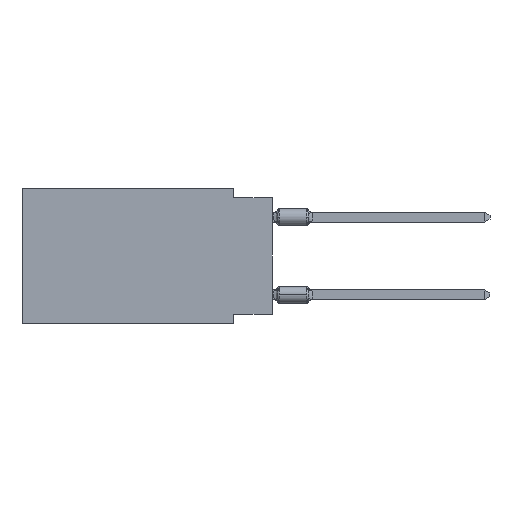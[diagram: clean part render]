
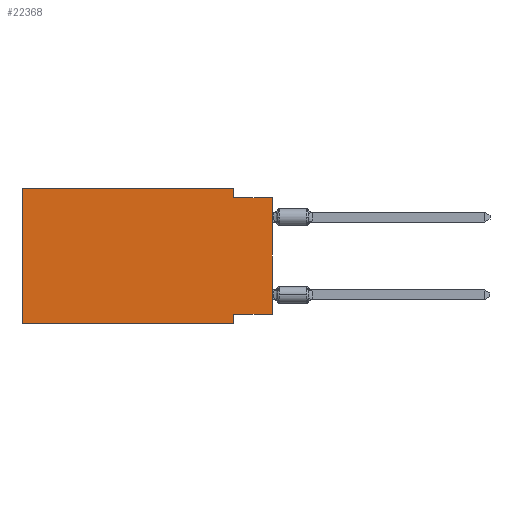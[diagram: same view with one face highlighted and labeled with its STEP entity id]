
A CAD part, left-side view. The second image highlights one B-rep face of the part: STEP entity #22368.
In plain terms, the highlighted planar face has unit normal (-1, 0, 0).
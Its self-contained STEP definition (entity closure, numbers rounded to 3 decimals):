
#188 = DIRECTION ( 'NONE',  ( 0., 0., 1. ) ) ;
#554 = PLANE ( 'NONE',  #14578 ) ;
#689 = CARTESIAN_POINT ( 'NONE',  ( 0., 16.383, -8.89 ) ) ;
#827 = ORIENTED_EDGE ( 'NONE', *, *, #16635, .F. ) ;
#1138 = DIRECTION ( 'NONE',  ( 0., -1., 0. ) ) ;
#1493 = VECTOR ( 'NONE', #17052, 1000. ) ;
#1579 = CARTESIAN_POINT ( 'NONE',  ( 0., 16.383, 0. ) ) ;
#1986 = ORIENTED_EDGE ( 'NONE', *, *, #21141, .F. ) ;
#2178 = FACE_OUTER_BOUND ( 'NONE', #10712, .T. ) ;
#2858 = ORIENTED_EDGE ( 'NONE', *, *, #10344, .F. ) ;
#2995 = EDGE_CURVE ( 'NONE', #13982, #20071, #6678, .T. ) ;
#3423 = VECTOR ( 'NONE', #1138, 1000. ) ;
#3777 = CARTESIAN_POINT ( 'NONE',  ( 0., 0., -8.255 ) ) ;
#3821 = DIRECTION ( 'NONE',  ( 1., 0., 0. ) ) ;
#3848 = CARTESIAN_POINT ( 'NONE',  ( 0., 2.54, -8.89 ) ) ;
#3850 = EDGE_CURVE ( 'NONE', #12104, #13905, #4719, .T. ) ;
#3902 = DIRECTION ( 'NONE',  ( 0., 0., 1. ) ) ;
#4116 = VECTOR ( 'NONE', #3902, 1000. ) ;
#4665 = LINE ( 'NONE', #18577, #15156 ) ;
#4695 = CARTESIAN_POINT ( 'NONE',  ( 0., 2.54, 0. ) ) ;
#4719 = LINE ( 'NONE', #20967, #14611 ) ;
#5555 = ORIENTED_EDGE ( 'NONE', *, *, #21640, .F. ) ;
#6438 = LINE ( 'NONE', #10158, #1493 ) ;
#6678 = LINE ( 'NONE', #17410, #22055 ) ;
#7951 = ORIENTED_EDGE ( 'NONE', *, *, #3850, .T. ) ;
#8048 = VERTEX_POINT ( 'NONE', #12262 ) ;
#8264 = CARTESIAN_POINT ( 'NONE',  ( 0., 0., -0.635 ) ) ;
#8575 = DIRECTION ( 'NONE',  ( 0., -1., 0. ) ) ;
#9146 = LINE ( 'NONE', #3777, #13728 ) ;
#9916 = DIRECTION ( 'NONE',  ( 0., 0., -1. ) ) ;
#10002 = LINE ( 'NONE', #8264, #3423 ) ;
#10158 = CARTESIAN_POINT ( 'NONE',  ( 0., 2.54, -8.89 ) ) ;
#10344 = EDGE_CURVE ( 'NONE', #20071, #12624, #4665, .T. ) ;
#10712 = EDGE_LOOP ( 'NONE', ( #11219, #827, #2858, #13090, #1986, #7951, #5555, #19471 ) ) ;
#10894 = DIRECTION ( 'NONE',  ( 0., 1., 0. ) ) ;
#10935 = DIRECTION ( 'NONE',  ( 0., 0., -1. ) ) ;
#11154 = EDGE_CURVE ( 'NONE', #11251, #8048, #9146, .T. ) ;
#11219 = ORIENTED_EDGE ( 'NONE', *, *, #22249, .T. ) ;
#11251 = VERTEX_POINT ( 'NONE', #11814 ) ;
#11814 = CARTESIAN_POINT ( 'NONE',  ( 0., 0., -8.255 ) ) ;
#12104 = VERTEX_POINT ( 'NONE', #689 ) ;
#12262 = CARTESIAN_POINT ( 'NONE',  ( 0., 2.54, -8.255 ) ) ;
#12624 = VERTEX_POINT ( 'NONE', #19704 ) ;
#12801 = LINE ( 'NONE', #21813, #16434 ) ;
#13090 = ORIENTED_EDGE ( 'NONE', *, *, #2995, .F. ) ;
#13728 = VECTOR ( 'NONE', #10894, 1000. ) ;
#13905 = VERTEX_POINT ( 'NONE', #3848 ) ;
#13982 = VERTEX_POINT ( 'NONE', #1579 ) ;
#14578 = AXIS2_PLACEMENT_3D ( 'NONE', #19829, #3821, #10935 ) ;
#14611 = VECTOR ( 'NONE', #8575, 1000. ) ;
#14754 = CARTESIAN_POINT ( 'NONE',  ( 0., 16.383, 0. ) ) ;
#14899 = CARTESIAN_POINT ( 'NONE',  ( 0., 0., -0.635 ) ) ;
#15156 = VECTOR ( 'NONE', #9916, 1000. ) ;
#16434 = VECTOR ( 'NONE', #188, 1000. ) ;
#16635 = EDGE_CURVE ( 'NONE', #12624, #18097, #10002, .T. ) ;
#17052 = DIRECTION ( 'NONE',  ( 0., 0., -1. ) ) ;
#17071 = DIRECTION ( 'NONE',  ( 0., -1., 0. ) ) ;
#17410 = CARTESIAN_POINT ( 'NONE',  ( 0., 16.383, 0. ) ) ;
#18097 = VERTEX_POINT ( 'NONE', #14899 ) ;
#18577 = CARTESIAN_POINT ( 'NONE',  ( 0., 2.54, 0. ) ) ;
#19471 = ORIENTED_EDGE ( 'NONE', *, *, #11154, .F. ) ;
#19704 = CARTESIAN_POINT ( 'NONE',  ( 0., 2.54, -0.635 ) ) ;
#19829 = CARTESIAN_POINT ( 'NONE',  ( 0., 16.383, 0. ) ) ;
#20071 = VERTEX_POINT ( 'NONE', #4695 ) ;
#20967 = CARTESIAN_POINT ( 'NONE',  ( 0., 16.383, -8.89 ) ) ;
#21141 = EDGE_CURVE ( 'NONE', #12104, #13982, #22139, .T. ) ;
#21640 = EDGE_CURVE ( 'NONE', #8048, #13905, #6438, .T. ) ;
#21813 = CARTESIAN_POINT ( 'NONE',  ( 0., 0., 0. ) ) ;
#22055 = VECTOR ( 'NONE', #17071, 1000. ) ;
#22139 = LINE ( 'NONE', #14754, #4116 ) ;
#22249 = EDGE_CURVE ( 'NONE', #11251, #18097, #12801, .T. ) ;
#22368 = ADVANCED_FACE ( 'NONE', ( #2178 ), #554, .F. ) ;
